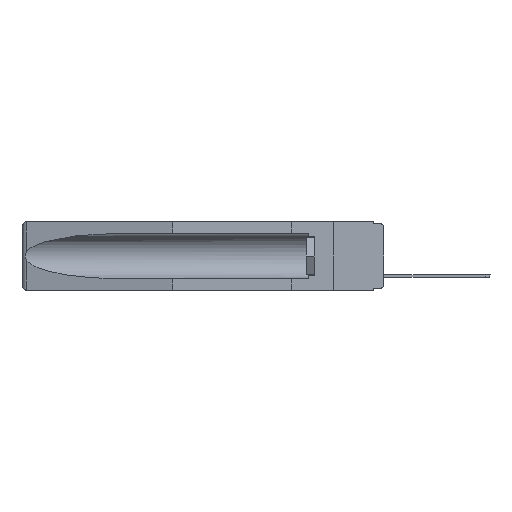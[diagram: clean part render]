
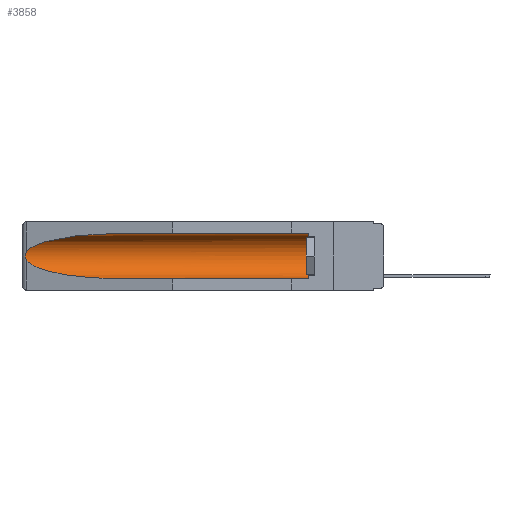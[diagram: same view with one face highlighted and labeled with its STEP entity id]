
A CAD part, left-side view. The second image highlights one B-rep face of the part: STEP entity #3858.
In plain terms, the highlighted cylindrical face has radius 2.857 mm (diameter 5.715 mm), a partial arc.
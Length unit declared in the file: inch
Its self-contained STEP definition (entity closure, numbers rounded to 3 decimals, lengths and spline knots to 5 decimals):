
#70 = CARTESIAN_POINT ( 'NONE',  ( 0.26537, 1.52718, -0.14972 ) ) ;
#219 = CARTESIAN_POINT ( 'NONE',  ( 0.26655, 1.53094, -0.18657 ) ) ;
#689 = ORIENTED_EDGE ( 'NONE', *, *, #7776, .T. ) ;
#900 = CARTESIAN_POINT ( 'NONE',  ( 0.155, -0.30754, -0.284 ) ) ;
#1052 = CARTESIAN_POINT ( 'NONE',  ( 0.21114, 1.30732, -0.284 ) ) ;
#1539 =( BOUNDED_CURVE ( )  B_SPLINE_CURVE ( 3, ( #24482, #3008, #1052, #13935 ),
 .UNSPECIFIED., .F., .T. ) 
 B_SPLINE_CURVE_WITH_KNOTS ( ( 4, 4 ),
 ( 0.1948, 1.5708 ),
 .UNSPECIFIED. ) 
 CURVE ( )  GEOMETRIC_REPRESENTATION_ITEM ( )  RATIONAL_B_SPLINE_CURVE ( ( 1., 0.848, 0.848, 1. ) ) 
 REPRESENTATION_ITEM ( '' )  );
#2572 = AXIS2_PLACEMENT_3D ( 'NONE', #2938, #9450, #4883 ) ;
#2938 = CARTESIAN_POINT ( 'NONE',  ( 0.155, 0.126, -0.1715 ) ) ;
#3008 = CARTESIAN_POINT ( 'NONE',  ( 0.25451, 1.48313, -0.24835 ) ) ;
#3560 = AXIS2_PLACEMENT_3D ( 'NONE', #22045, #26879, #11506 ) ;
#3777 = CARTESIAN_POINT ( 'NONE',  ( 0.155, 1.07973, -0.059 ) ) ;
#3858 = ADVANCED_FACE ( 'NONE', ( #22177 ), #15922, .F. ) ;
#4397 = CARTESIAN_POINT ( 'NONE',  ( 0.26654, 1.53092, -0.15636 ) ) ;
#4883 = DIRECTION ( 'NONE',  ( 0., 0., 1. ) ) ;
#5266 = CARTESIAN_POINT ( 'NONE',  ( 0.21114, 1.30732, -0.059 ) ) ;
#5742 = CARTESIAN_POINT ( 'NONE',  ( 0.155, -0.30754, -0.059 ) ) ;
#6047 = ORIENTED_EDGE ( 'NONE', *, *, #8878, .F. ) ;
#6497 = DIRECTION ( 'NONE',  ( 0., 1., 0. ) ) ;
#6514 = VERTEX_POINT ( 'NONE', #3777 ) ;
#7192 = CARTESIAN_POINT ( 'NONE',  ( 0.155, 1.07973, -0.284 ) ) ;
#7293 = LINE ( 'NONE', #900, #20049 ) ;
#7480 = VERTEX_POINT ( 'NONE', #23237 ) ;
#7581 = VERTEX_POINT ( 'NONE', #70 ) ;
#7776 = EDGE_CURVE ( 'NONE', #14179, #6514, #20572, .T. ) ;
#8878 = EDGE_CURVE ( 'NONE', #7480, #16268, #7293, .T. ) ;
#9173 = EDGE_LOOP ( 'NONE', ( #9458, #12403, #20076, #6047, #13913, #689 ) ) ;
#9450 = DIRECTION ( 'NONE',  ( 0., -1., 0. ) ) ;
#9458 = ORIENTED_EDGE ( 'NONE', *, *, #23272, .T. ) ;
#9905 = DIRECTION ( 'NONE',  ( 0., 1., 0. ) ) ;
#10351 = CARTESIAN_POINT ( 'NONE',  ( 0.2675, 1.53308, -0.16763 ) ) ;
#11506 = DIRECTION ( 'NONE',  ( 0., 0., 1. ) ) ;
#11776 = EDGE_CURVE ( 'NONE', #7581, #22616, #19249, .T. ) ;
#12403 = ORIENTED_EDGE ( 'NONE', *, *, #11776, .T. ) ;
#12429 = CARTESIAN_POINT ( 'NONE',  ( 0.2673, 1.5327, -0.16383 ) ) ;
#13913 = ORIENTED_EDGE ( 'NONE', *, *, #18830, .T. ) ;
#13935 = CARTESIAN_POINT ( 'NONE',  ( 0.155, 1.07973, -0.284 ) ) ;
#14179 = VERTEX_POINT ( 'NONE', #20931 ) ;
#14498 = CARTESIAN_POINT ( 'NONE',  ( 0.26537, 1.52718, -0.14972 ) ) ;
#15043 = VECTOR ( 'NONE', #9905, 39.37008 ) ;
#15922 = CYLINDRICAL_SURFACE ( 'NONE', #3560, 0.1125 ) ;
#16035 =( BOUNDED_CURVE ( )  B_SPLINE_CURVE ( 3, ( #22044, #5266, #21916, #20353 ),
 .UNSPECIFIED., .F., .T. ) 
 B_SPLINE_CURVE_WITH_KNOTS ( ( 4, 4 ),
 ( 4.71239, 6.08839 ),
 .UNSPECIFIED. ) 
 CURVE ( )  GEOMETRIC_REPRESENTATION_ITEM ( )  RATIONAL_B_SPLINE_CURVE ( ( 1., 0.848, 0.848, 1. ) ) 
 REPRESENTATION_ITEM ( '' )  );
#16268 = VERTEX_POINT ( 'NONE', #7192 ) ;
#17129 = CARTESIAN_POINT ( 'NONE',  ( 0.2673, 1.53269, -0.17917 ) ) ;
#18375 = CARTESIAN_POINT ( 'NONE',  ( 0.26537, 1.52718, -0.19328 ) ) ;
#18793 = CARTESIAN_POINT ( 'NONE',  ( 0.2675, 1.53308, -0.17534 ) ) ;
#18830 = EDGE_CURVE ( 'NONE', #7480, #14179, #20276, .T. ) ;
#19249 = B_SPLINE_CURVE_WITH_KNOTS ( 'NONE', 3,
 ( #14498, #23385, #4397, #12429, #10351, #18793, #17129, #219, #25602, #25740 ),
 .UNSPECIFIED., .F., .F.,
 ( 4, 2, 2, 2, 4 ),
 ( 0., 0.00029, 0.00058, 0.00087, 0.00117 ),
 .UNSPECIFIED. ) ;
#19343 = EDGE_CURVE ( 'NONE', #22616, #16268, #1539, .T. ) ;
#20049 = VECTOR ( 'NONE', #6497, 39.37008 ) ;
#20076 = ORIENTED_EDGE ( 'NONE', *, *, #19343, .T. ) ;
#20276 = CIRCLE ( 'NONE', #2572, 0.1125 ) ;
#20353 = CARTESIAN_POINT ( 'NONE',  ( 0.26537, 1.52718, -0.14972 ) ) ;
#20572 = LINE ( 'NONE', #5742, #15043 ) ;
#20931 = CARTESIAN_POINT ( 'NONE',  ( 0.155, 0.126, -0.059 ) ) ;
#21916 = CARTESIAN_POINT ( 'NONE',  ( 0.25451, 1.48313, -0.09465 ) ) ;
#22044 = CARTESIAN_POINT ( 'NONE',  ( 0.155, 1.07973, -0.059 ) ) ;
#22045 = CARTESIAN_POINT ( 'NONE',  ( 0.155, -0.30754, -0.1715 ) ) ;
#22177 = FACE_OUTER_BOUND ( 'NONE', #9173, .T. ) ;
#22616 = VERTEX_POINT ( 'NONE', #18375 ) ;
#23237 = CARTESIAN_POINT ( 'NONE',  ( 0.155, 0.126, -0.284 ) ) ;
#23272 = EDGE_CURVE ( 'NONE', #6514, #7581, #16035, .T. ) ;
#23385 = CARTESIAN_POINT ( 'NONE',  ( 0.26597, 1.52961, -0.15275 ) ) ;
#24482 = CARTESIAN_POINT ( 'NONE',  ( 0.26537, 1.52718, -0.19328 ) ) ;
#25602 = CARTESIAN_POINT ( 'NONE',  ( 0.26597, 1.5296, -0.19026 ) ) ;
#25740 = CARTESIAN_POINT ( 'NONE',  ( 0.26537, 1.52718, -0.19328 ) ) ;
#26879 = DIRECTION ( 'NONE',  ( 0., 1., 0. ) ) ;
